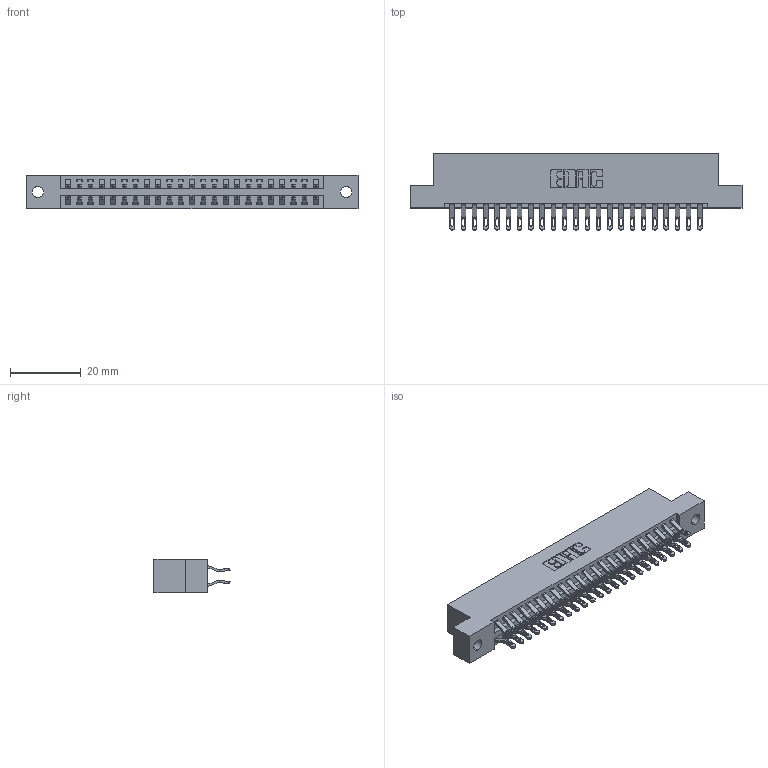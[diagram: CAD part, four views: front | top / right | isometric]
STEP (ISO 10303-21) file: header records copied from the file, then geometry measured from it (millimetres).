
FILE_DESCRIPTION (( 'STEP AP203' ), '1' );
FILE_NAME ('346-046-555-202.STEP', '2018-08-25T06:11:00', ( '' ), ( '' ), 'SwSTEP 2.0', 'SolidWorks 2016', '' );
FILE_SCHEMA (( 'CONFIG_CONTROL_DESIGN' ));
Length unit declared in the file: inch
Products named in the file (3): 346 Part_Flush Mounting Lugs - 0.128 Dia; 345-292-001_555 Tail; 346-046-555-202
Assembly tree (47 placements, depth 2):
  346-046-555-202
    346 Part_Flush Mounting Lugs - 0.128 Dia
    345-292-001_555 Tail  x46
Bounding box: 93.6 x 21.46 x 9.4 mm (x, y, z)
Volume: 9076.2 mm3; surface area: 12383.6 mm2
Topology: 47 solids, 47 shells, 2790 faces, 8747 edges, 5830 vertices
Faces by surface type: plane 1594, cylinder 1196
Entity records: 17897 total; most frequent: CARTESIAN_POINT 3010, ORIENTED_EDGE 2914, DIRECTION 2673, EDGE_CURVE 1457, LINE 1213, VECTOR 1213, VERTEX_POINT 970, AXIS2_PLACEMENT_3D 730
